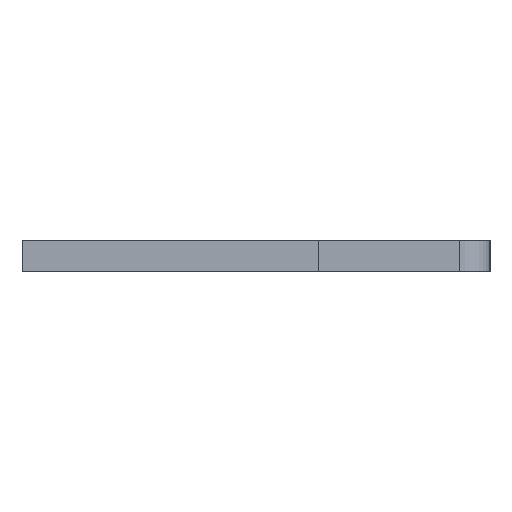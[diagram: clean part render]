
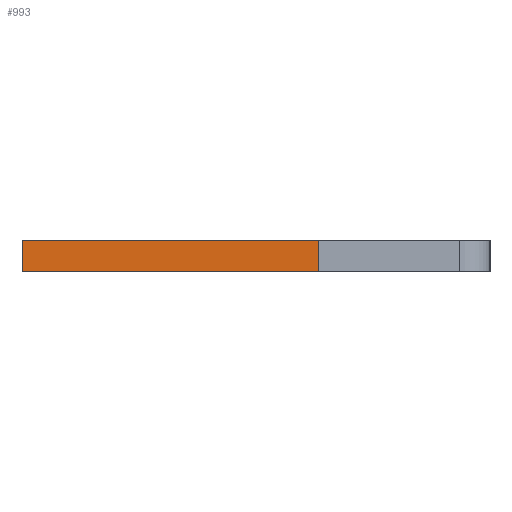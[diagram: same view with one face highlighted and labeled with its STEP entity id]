
A CAD part, left-side view. The second image highlights one B-rep face of the part: STEP entity #993.
In plain terms, the highlighted face is planar.
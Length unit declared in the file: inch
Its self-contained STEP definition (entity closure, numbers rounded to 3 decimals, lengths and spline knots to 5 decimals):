
#24 = DIRECTION ( 'NONE',  ( 0., 1., 0. ) ) ;
#48 = DIRECTION ( 'NONE',  ( -1., 0., 0. ) ) ;
#61 = VERTEX_POINT ( 'NONE', #201 ) ;
#128 = LINE ( 'NONE', #414, #1002 ) ;
#142 = CARTESIAN_POINT ( 'NONE',  ( 0.01, 0.15, -0.04 ) ) ;
#199 = VERTEX_POINT ( 'NONE', #599 ) ;
#201 = CARTESIAN_POINT ( 'NONE',  ( 0.01, -0.04, -0.04 ) ) ;
#202 = VERTEX_POINT ( 'NONE', #852 ) ;
#220 = VECTOR ( 'NONE', #24, 39.37008 ) ;
#399 = DIRECTION ( 'NONE',  ( 0., 1., 0. ) ) ;
#414 = CARTESIAN_POINT ( 'NONE',  ( 0.01, -0.04, -0.04 ) ) ;
#476 = VECTOR ( 'NONE', #48, 39.37008 ) ;
#527 = EDGE_CURVE ( 'NONE', #61, #1467, #625, .T. ) ;
#535 = CARTESIAN_POINT ( 'NONE',  ( 0.01, 0.15, -0.04 ) ) ;
#599 = CARTESIAN_POINT ( 'NONE',  ( -0.01, -0.04, -0.04 ) ) ;
#625 = LINE ( 'NONE', #142, #220 ) ;
#737 = EDGE_CURVE ( 'NONE', #199, #202, #1148, .T. ) ;
#852 = CARTESIAN_POINT ( 'NONE',  ( -0.01, 0.15, -0.04 ) ) ;
#915 = DIRECTION ( 'NONE',  ( 1., 0., 0. ) ) ;
#922 = VECTOR ( 'NONE', #399, 39.37008 ) ;
#937 = ORIENTED_EDGE ( 'NONE', *, *, #962, .T. ) ;
#962 = EDGE_CURVE ( 'NONE', #61, #199, #128, .T. ) ;
#993 = ADVANCED_FACE ( 'NONE', ( #1205 ), #1050, .F. ) ;
#1002 = VECTOR ( 'NONE', #1275, 39.37008 ) ;
#1050 = PLANE ( 'NONE',  #1310 ) ;
#1135 = CARTESIAN_POINT ( 'NONE',  ( -0.01, 0.15, -0.04 ) ) ;
#1148 = LINE ( 'NONE', #1135, #922 ) ;
#1160 = EDGE_LOOP ( 'NONE', ( #1417, #1219, #1426, #937 ) ) ;
#1189 = CARTESIAN_POINT ( 'NONE',  ( 0.01, 0.15, -0.04 ) ) ;
#1198 = EDGE_CURVE ( 'NONE', #1467, #202, #1430, .T. ) ;
#1205 = FACE_OUTER_BOUND ( 'NONE', #1160, .T. ) ;
#1219 = ORIENTED_EDGE ( 'NONE', *, *, #1198, .F. ) ;
#1275 = DIRECTION ( 'NONE',  ( -1., 0., 0. ) ) ;
#1310 = AXIS2_PLACEMENT_3D ( 'NONE', #535, #1505, #915 ) ;
#1417 = ORIENTED_EDGE ( 'NONE', *, *, #737, .T. ) ;
#1426 = ORIENTED_EDGE ( 'NONE', *, *, #527, .F. ) ;
#1430 = LINE ( 'NONE', #1514, #476 ) ;
#1467 = VERTEX_POINT ( 'NONE', #1189 ) ;
#1505 = DIRECTION ( 'NONE',  ( 0., 0., 1. ) ) ;
#1514 = CARTESIAN_POINT ( 'NONE',  ( 0.01, 0.15, -0.04 ) ) ;
